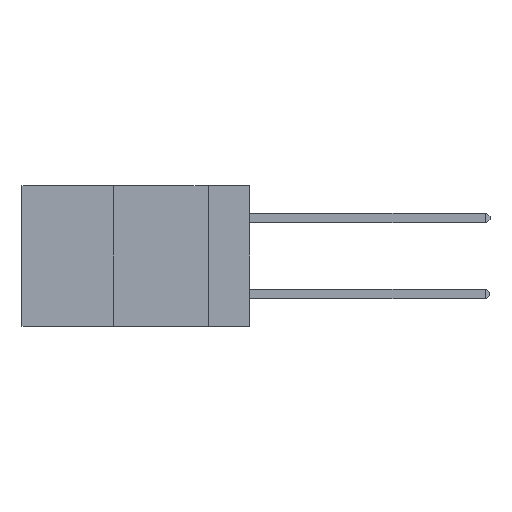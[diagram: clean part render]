
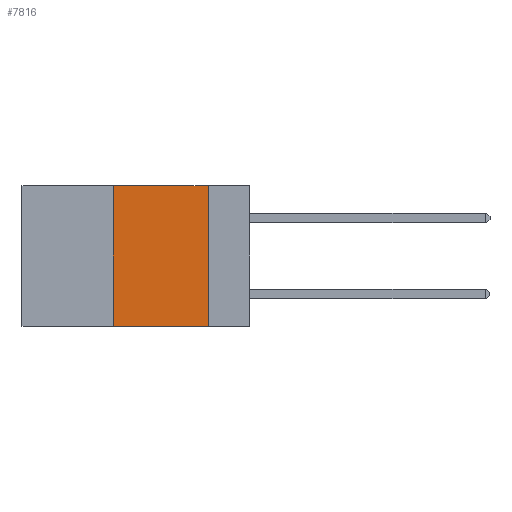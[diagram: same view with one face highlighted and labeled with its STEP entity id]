
A CAD part, left-side view. The second image highlights one B-rep face of the part: STEP entity #7816.
In plain terms, the highlighted planar face has unit normal (-1, 0, 0).
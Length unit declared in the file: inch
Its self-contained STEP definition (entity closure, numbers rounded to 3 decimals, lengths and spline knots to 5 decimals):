
#273 = VERTEX_POINT ( 'NONE', #6424 ) ;
#419 = CARTESIAN_POINT ( 'NONE',  ( 0., 0.6, 0. ) ) ;
#514 = EDGE_CURVE ( 'NONE', #875, #2047, #4378, .T. ) ;
#674 = FACE_OUTER_BOUND ( 'NONE', #851, .T. ) ;
#851 = EDGE_LOOP ( 'NONE', ( #2645, #2739, #3608, #3622 ) ) ;
#875 = VERTEX_POINT ( 'NONE', #3186 ) ;
#881 = CARTESIAN_POINT ( 'NONE',  ( 0., 0.6, 0. ) ) ;
#1931 = LINE ( 'NONE', #9430, #5877 ) ;
#2047 = VERTEX_POINT ( 'NONE', #9585 ) ;
#2139 = PLANE ( 'NONE',  #4312 ) ;
#2645 = ORIENTED_EDGE ( 'NONE', *, *, #5576, .F. ) ;
#2739 = ORIENTED_EDGE ( 'NONE', *, *, #514, .F. ) ;
#2958 = DIRECTION ( 'NONE',  ( 1., 0., 0. ) ) ;
#3186 = CARTESIAN_POINT ( 'NONE',  ( 0., 0.36, 0. ) ) ;
#3359 = VECTOR ( 'NONE', #9075, 39.37008 ) ;
#3608 = ORIENTED_EDGE ( 'NONE', *, *, #6095, .F. ) ;
#3622 = ORIENTED_EDGE ( 'NONE', *, *, #8899, .T. ) ;
#4312 = AXIS2_PLACEMENT_3D ( 'NONE', #419, #2958, #8120 ) ;
#4378 = LINE ( 'NONE', #881, #6136 ) ;
#4628 = CARTESIAN_POINT ( 'NONE',  ( 0., 0.6, -0.37 ) ) ;
#4674 = CARTESIAN_POINT ( 'NONE',  ( 0., 0.36, 0. ) ) ;
#5013 = CARTESIAN_POINT ( 'NONE',  ( 0., 0.11, -0.37 ) ) ;
#5329 = VECTOR ( 'NONE', #8902, 39.37008 ) ;
#5566 = DIRECTION ( 'NONE',  ( 0., -1., 0. ) ) ;
#5576 = EDGE_CURVE ( 'NONE', #2047, #9285, #1931, .T. ) ;
#5877 = VECTOR ( 'NONE', #8797, 39.37008 ) ;
#6095 = EDGE_CURVE ( 'NONE', #273, #875, #9078, .T. ) ;
#6136 = VECTOR ( 'NONE', #5566, 39.37008 ) ;
#6424 = CARTESIAN_POINT ( 'NONE',  ( 0., 0.36, -0.37 ) ) ;
#7470 = LINE ( 'NONE', #4628, #5329 ) ;
#7816 = ADVANCED_FACE ( 'NONE', ( #674 ), #2139, .F. ) ;
#8120 = DIRECTION ( 'NONE',  ( 0., 0., -1. ) ) ;
#8797 = DIRECTION ( 'NONE',  ( 0., 0., -1. ) ) ;
#8899 = EDGE_CURVE ( 'NONE', #273, #9285, #7470, .T. ) ;
#8902 = DIRECTION ( 'NONE',  ( 0., -1., 0. ) ) ;
#9075 = DIRECTION ( 'NONE',  ( 0., 0., 1. ) ) ;
#9078 = LINE ( 'NONE', #4674, #3359 ) ;
#9285 = VERTEX_POINT ( 'NONE', #5013 ) ;
#9430 = CARTESIAN_POINT ( 'NONE',  ( 0., 0.11, 0. ) ) ;
#9585 = CARTESIAN_POINT ( 'NONE',  ( 0., 0.11, 0. ) ) ;
